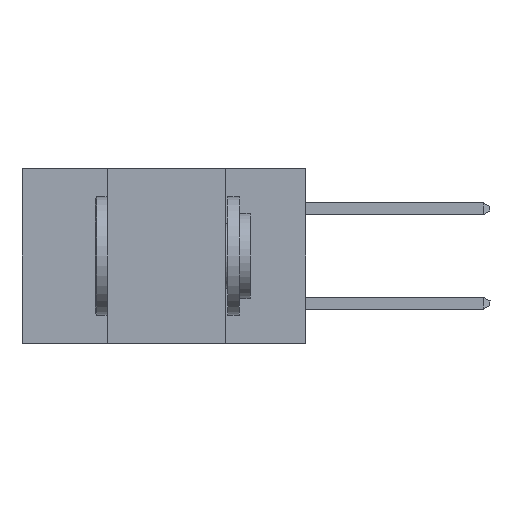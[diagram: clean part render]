
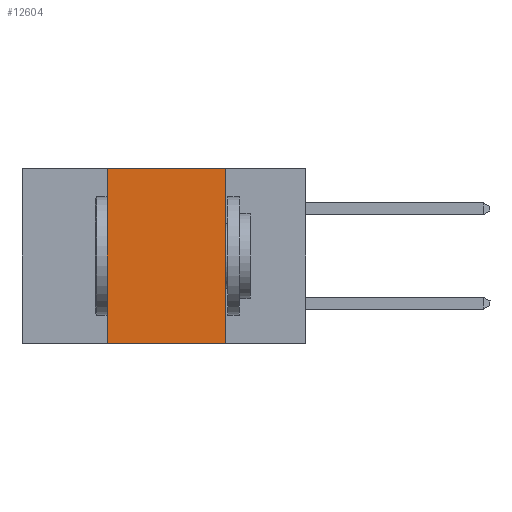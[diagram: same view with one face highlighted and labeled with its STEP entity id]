
A CAD part, left-side view. The second image highlights one B-rep face of the part: STEP entity #12604.
In plain terms, the highlighted planar face has unit normal (-1, 0, 0).
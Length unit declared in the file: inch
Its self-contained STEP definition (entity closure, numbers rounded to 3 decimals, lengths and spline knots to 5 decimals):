
#349 = AXIS2_PLACEMENT_3D ( 'NONE', #2197, #1870, #1707 ) ;
#575 = LINE ( 'NONE', #13651, #10310 ) ;
#680 = CARTESIAN_POINT ( 'NONE',  ( 0., 0.42, -0.37 ) ) ;
#699 = VERTEX_POINT ( 'NONE', #11332 ) ;
#847 = VERTEX_POINT ( 'NONE', #10150 ) ;
#1707 = DIRECTION ( 'NONE',  ( 0., 0., -1. ) ) ;
#1870 = DIRECTION ( 'NONE',  ( 1., 0., 0. ) ) ;
#1969 = PLANE ( 'NONE',  #349 ) ;
#2197 = CARTESIAN_POINT ( 'NONE',  ( 0., 0.6, 0. ) ) ;
#2796 = LINE ( 'NONE', #11590, #15895 ) ;
#3187 = FACE_OUTER_BOUND ( 'NONE', #6419, .T. ) ;
#4906 = ORIENTED_EDGE ( 'NONE', *, *, #13005, .F. ) ;
#5146 = VERTEX_POINT ( 'NONE', #680 ) ;
#5477 = ORIENTED_EDGE ( 'NONE', *, *, #10544, .T. ) ;
#6419 = EDGE_LOOP ( 'NONE', ( #10478, #4906, #11640, #5477 ) ) ;
#7002 = DIRECTION ( 'NONE',  ( 0., 0., -1. ) ) ;
#7024 = CARTESIAN_POINT ( 'NONE',  ( 0., 0.17, -0.37 ) ) ;
#7858 = DIRECTION ( 'NONE',  ( 0., -1., 0. ) ) ;
#8272 = CARTESIAN_POINT ( 'NONE',  ( 0., 0.6, -0.37 ) ) ;
#9461 = VECTOR ( 'NONE', #7002, 39.37008 ) ;
#9867 = LINE ( 'NONE', #7024, #9461 ) ;
#10150 = CARTESIAN_POINT ( 'NONE',  ( 0., 0.42, 0. ) ) ;
#10310 = VECTOR ( 'NONE', #13665, 39.37008 ) ;
#10478 = ORIENTED_EDGE ( 'NONE', *, *, #13791, .F. ) ;
#10544 = EDGE_CURVE ( 'NONE', #5146, #699, #12862, .T. ) ;
#10962 = VERTEX_POINT ( 'NONE', #15160 ) ;
#11332 = CARTESIAN_POINT ( 'NONE',  ( 0., 0.17, -0.37 ) ) ;
#11582 = DIRECTION ( 'NONE',  ( 0., 0., 1. ) ) ;
#11590 = CARTESIAN_POINT ( 'NONE',  ( 0., 0.42, -0.37 ) ) ;
#11640 = ORIENTED_EDGE ( 'NONE', *, *, #12178, .F. ) ;
#12178 = EDGE_CURVE ( 'NONE', #5146, #847, #2796, .T. ) ;
#12452 = VECTOR ( 'NONE', #7858, 39.37008 ) ;
#12604 = ADVANCED_FACE ( 'NONE', ( #3187 ), #1969, .F. ) ;
#12862 = LINE ( 'NONE', #8272, #12452 ) ;
#13005 = EDGE_CURVE ( 'NONE', #847, #10962, #575, .T. ) ;
#13651 = CARTESIAN_POINT ( 'NONE',  ( 0., 0.6, 0. ) ) ;
#13665 = DIRECTION ( 'NONE',  ( 0., -1., 0. ) ) ;
#13791 = EDGE_CURVE ( 'NONE', #10962, #699, #9867, .T. ) ;
#15160 = CARTESIAN_POINT ( 'NONE',  ( 0., 0.17, 0. ) ) ;
#15895 = VECTOR ( 'NONE', #11582, 39.37008 ) ;
